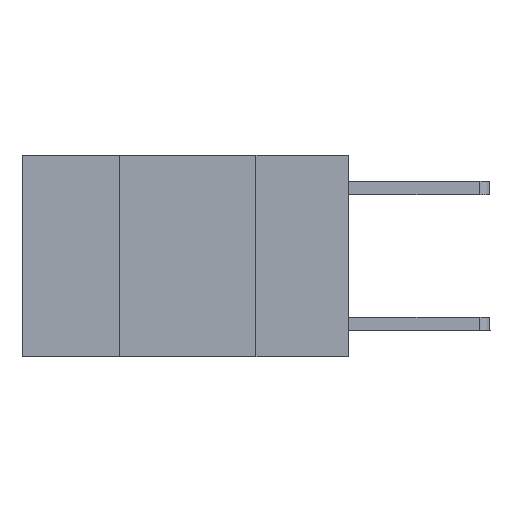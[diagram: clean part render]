
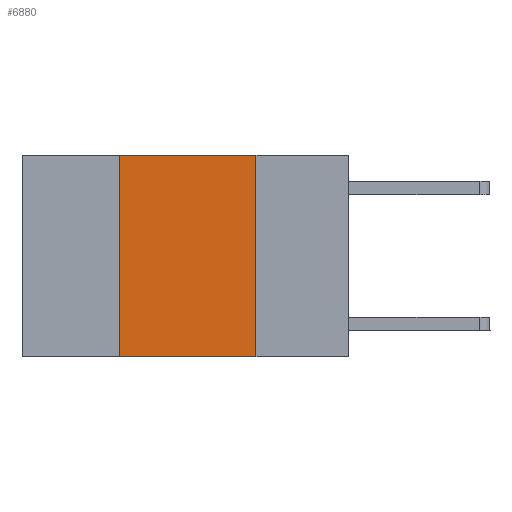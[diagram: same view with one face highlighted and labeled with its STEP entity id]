
A CAD part, left-side view. The second image highlights one B-rep face of the part: STEP entity #6880.
In plain terms, the highlighted planar face has unit normal (-1, 0, 0).
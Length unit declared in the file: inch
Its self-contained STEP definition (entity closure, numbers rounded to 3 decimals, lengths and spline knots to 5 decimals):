
#299 = EDGE_LOOP ( 'NONE', ( #3964, #4001, #4020, #4120 ) ) ;
#473 = VECTOR ( 'NONE', #7438, 39.37008 ) ;
#573 = CARTESIAN_POINT ( 'NONE',  ( 0., 0.42, 0. ) ) ;
#687 = DIRECTION ( 'NONE',  ( 0., 0., 1. ) ) ;
#1054 = VERTEX_POINT ( 'NONE', #9899 ) ;
#1135 = PLANE ( 'NONE',  #10678 ) ;
#1160 = LINE ( 'NONE', #4054, #9627 ) ;
#1269 = EDGE_CURVE ( 'NONE', #1759, #1054, #9408, .T. ) ;
#1759 = VERTEX_POINT ( 'NONE', #4788 ) ;
#2787 = LINE ( 'NONE', #6597, #473 ) ;
#3252 = EDGE_CURVE ( 'NONE', #7855, #1759, #10506, .T. ) ;
#3964 = ORIENTED_EDGE ( 'NONE', *, *, #9961, .F. ) ;
#4001 = ORIENTED_EDGE ( 'NONE', *, *, #1269, .F. ) ;
#4020 = ORIENTED_EDGE ( 'NONE', *, *, #3252, .F. ) ;
#4054 = CARTESIAN_POINT ( 'NONE',  ( 0., 0.17, 0. ) ) ;
#4088 = CARTESIAN_POINT ( 'NONE',  ( 0., 0.17, -0.37 ) ) ;
#4120 = ORIENTED_EDGE ( 'NONE', *, *, #5160, .T. ) ;
#4650 = DIRECTION ( 'NONE',  ( 1., 0., 0. ) ) ;
#4788 = CARTESIAN_POINT ( 'NONE',  ( 0., 0.42, 0. ) ) ;
#4994 = CARTESIAN_POINT ( 'NONE',  ( 0., 0.42, -0.37 ) ) ;
#5160 = EDGE_CURVE ( 'NONE', #7855, #9989, #2787, .T. ) ;
#5557 = CARTESIAN_POINT ( 'NONE',  ( 0., 0.6, 0. ) ) ;
#5959 = VECTOR ( 'NONE', #687, 39.37008 ) ;
#6597 = CARTESIAN_POINT ( 'NONE',  ( 0., 0.6, -0.37 ) ) ;
#6880 = ADVANCED_FACE ( 'NONE', ( #10308 ), #1135, .F. ) ;
#7438 = DIRECTION ( 'NONE',  ( 0., -1., 0. ) ) ;
#7855 = VERTEX_POINT ( 'NONE', #4994 ) ;
#8874 = DIRECTION ( 'NONE',  ( 0., -1., 0. ) ) ;
#9070 = DIRECTION ( 'NONE',  ( 0., 0., -1. ) ) ;
#9170 = VECTOR ( 'NONE', #8874, 39.37008 ) ;
#9408 = LINE ( 'NONE', #5557, #9170 ) ;
#9607 = CARTESIAN_POINT ( 'NONE',  ( 0., 0.6, 0. ) ) ;
#9627 = VECTOR ( 'NONE', #9070, 39.37008 ) ;
#9899 = CARTESIAN_POINT ( 'NONE',  ( 0., 0.17, 0. ) ) ;
#9961 = EDGE_CURVE ( 'NONE', #1054, #9989, #1160, .T. ) ;
#9989 = VERTEX_POINT ( 'NONE', #4088 ) ;
#10308 = FACE_OUTER_BOUND ( 'NONE', #299, .T. ) ;
#10377 = DIRECTION ( 'NONE',  ( 0., 0., -1. ) ) ;
#10506 = LINE ( 'NONE', #573, #5959 ) ;
#10678 = AXIS2_PLACEMENT_3D ( 'NONE', #9607, #4650, #10377 ) ;
